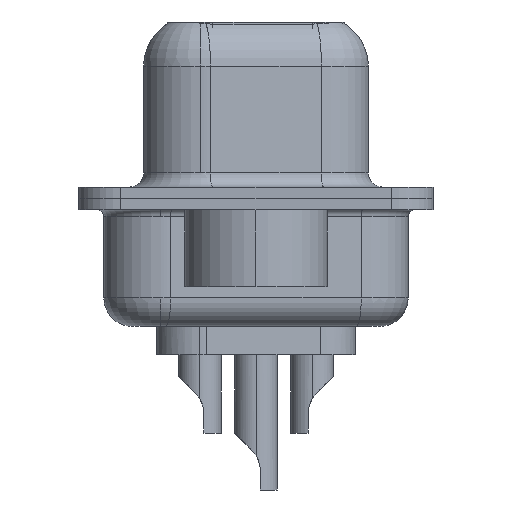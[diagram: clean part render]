
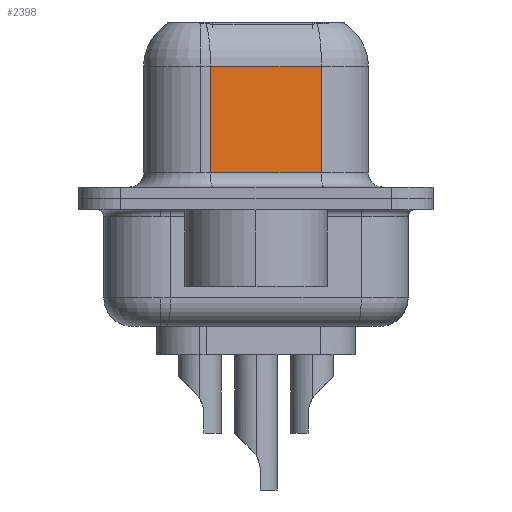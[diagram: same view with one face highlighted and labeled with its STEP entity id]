
A CAD part, left-side view. The second image highlights one B-rep face of the part: STEP entity #2398.
In plain terms, the highlighted planar face has unit normal (-0.985, -0.174, 0).
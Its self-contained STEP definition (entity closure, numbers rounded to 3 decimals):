
#750 = DIRECTION ( 'NONE',  ( 0., 0., -1. ) ) ;
#1518 = VECTOR ( 'NONE', #12019, 1000. ) ;
#2398 = ADVANCED_FACE ( 'NONE', ( #22462 ), #19681, .F. ) ;
#3176 = VECTOR ( 'NONE', #750, 1000. ) ;
#3383 = CARTESIAN_POINT ( 'NONE',  ( 4.355, 1.603, 6.4 ) ) ;
#3538 = DIRECTION ( 'NONE',  ( 0.174, -0.985, 0. ) ) ;
#3705 = VERTEX_POINT ( 'NONE', #22317 ) ;
#4446 = VECTOR ( 'NONE', #11618, 1000. ) ;
#5197 = DIRECTION ( 'NONE',  ( 0.985, 0.174, 0. ) ) ;
#5635 = DIRECTION ( 'NONE',  ( -0.174, 0.985, 0. ) ) ;
#6772 = CARTESIAN_POINT ( 'NONE',  ( 5.043, -2.297, 4.65 ) ) ;
#6857 = EDGE_CURVE ( 'NONE', #3705, #15386, #16688, .T. ) ;
#7038 = VECTOR ( 'NONE', #3538, 1000. ) ;
#7995 = EDGE_CURVE ( 'NONE', #30793, #8453, #8066, .T. ) ;
#8066 = LINE ( 'NONE', #3383, #3176 ) ;
#8453 = VERTEX_POINT ( 'NONE', #27382 ) ;
#8484 = ORIENTED_EDGE ( 'NONE', *, *, #6857, .F. ) ;
#9612 = ORIENTED_EDGE ( 'NONE', *, *, #19938, .T. ) ;
#11618 = DIRECTION ( 'NONE',  ( -0.174, 0.985, 0. ) ) ;
#12019 = DIRECTION ( 'NONE',  ( 0., 0., -1. ) ) ;
#13800 = AXIS2_PLACEMENT_3D ( 'NONE', #17788, #5197, #5635 ) ;
#13964 = LINE ( 'NONE', #6772, #4446 ) ;
#15386 = VERTEX_POINT ( 'NONE', #29307 ) ;
#16688 = LINE ( 'NONE', #23867, #1518 ) ;
#17788 = CARTESIAN_POINT ( 'NONE',  ( 5.043, -2.297, 6.4 ) ) ;
#19681 = PLANE ( 'NONE',  #13800 ) ;
#19856 = EDGE_LOOP ( 'NONE', ( #8484, #26616, #24018, #9612 ) ) ;
#19938 = EDGE_CURVE ( 'NONE', #8453, #15386, #27419, .T. ) ;
#22317 = CARTESIAN_POINT ( 'NONE',  ( 5.043, -2.297, 4.65 ) ) ;
#22462 = FACE_OUTER_BOUND ( 'NONE', #19856, .T. ) ;
#23867 = CARTESIAN_POINT ( 'NONE',  ( 5.043, -2.297, 6.4 ) ) ;
#24018 = ORIENTED_EDGE ( 'NONE', *, *, #7995, .T. ) ;
#25193 = CARTESIAN_POINT ( 'NONE',  ( 4.355, 1.603, 4.65 ) ) ;
#25724 = EDGE_CURVE ( 'NONE', #3705, #30793, #13964, .T. ) ;
#26616 = ORIENTED_EDGE ( 'NONE', *, *, #25724, .T. ) ;
#27382 = CARTESIAN_POINT ( 'NONE',  ( 4.355, 1.603, 0.9 ) ) ;
#27419 = LINE ( 'NONE', #29295, #7038 ) ;
#29295 = CARTESIAN_POINT ( 'NONE',  ( 5.043, -2.297, 0.9 ) ) ;
#29307 = CARTESIAN_POINT ( 'NONE',  ( 5.043, -2.297, 0.9 ) ) ;
#30793 = VERTEX_POINT ( 'NONE', #25193 ) ;
